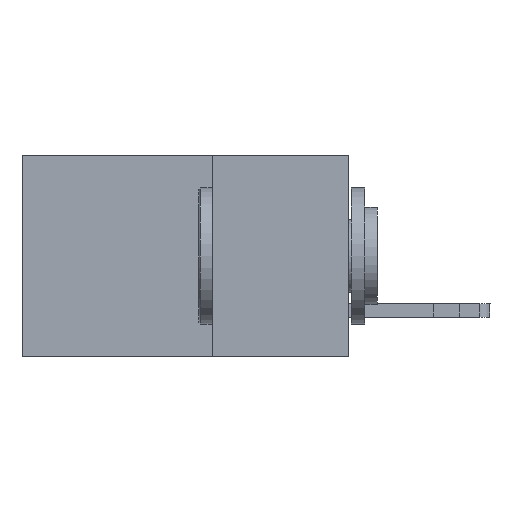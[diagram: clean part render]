
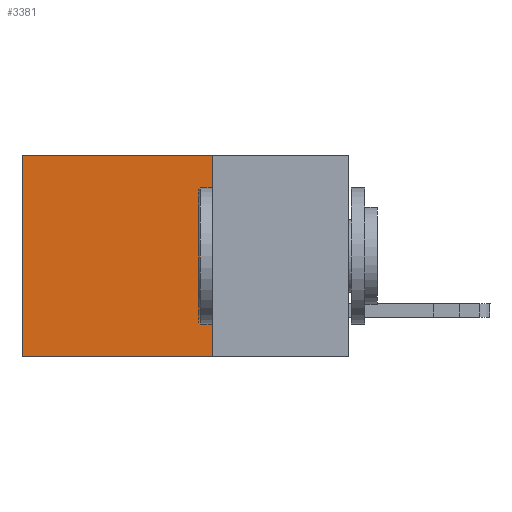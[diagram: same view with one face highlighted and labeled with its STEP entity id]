
A CAD part, left-side view. The second image highlights one B-rep face of the part: STEP entity #3381.
In plain terms, the highlighted planar face has unit normal (-1, 0, 0).
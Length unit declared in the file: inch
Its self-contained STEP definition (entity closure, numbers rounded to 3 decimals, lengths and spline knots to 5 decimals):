
#71 = CARTESIAN_POINT ( 'NONE',  ( 0.2615, 0.25, 0. ) ) ;
#159 = PLANE ( 'NONE',  #5733 ) ;
#172 = CARTESIAN_POINT ( 'NONE',  ( 0.2615, 0.25, -0.37 ) ) ;
#450 = ORIENTED_EDGE ( 'NONE', *, *, #9704, .T. ) ;
#469 = VERTEX_POINT ( 'NONE', #11647 ) ;
#1218 = VERTEX_POINT ( 'NONE', #1797 ) ;
#1279 = EDGE_LOOP ( 'NONE', ( #4782, #8911, #9141, #450 ) ) ;
#1305 = DIRECTION ( 'NONE',  ( 0., 0., -1. ) ) ;
#1797 = CARTESIAN_POINT ( 'NONE',  ( 0.2615, 0.25, -0.37 ) ) ;
#1915 = LINE ( 'NONE', #2898, #6736 ) ;
#2261 = LINE ( 'NONE', #172, #6209 ) ;
#2370 = DIRECTION ( 'NONE',  ( 0., 0., -1. ) ) ;
#2437 = VECTOR ( 'NONE', #9792, 39.37008 ) ;
#2898 = CARTESIAN_POINT ( 'NONE',  ( 0.2615, 0.6, -0.37 ) ) ;
#3381 = ADVANCED_FACE ( 'NONE', ( #3504 ), #159, .F. ) ;
#3504 = FACE_OUTER_BOUND ( 'NONE', #1279, .T. ) ;
#4010 = CARTESIAN_POINT ( 'NONE',  ( 0.2615, 0.6, 0. ) ) ;
#4064 = EDGE_CURVE ( 'NONE', #11904, #6744, #1915, .T. ) ;
#4187 = EDGE_CURVE ( 'NONE', #469, #1218, #2261, .T. ) ;
#4782 = ORIENTED_EDGE ( 'NONE', *, *, #4064, .T. ) ;
#5733 = AXIS2_PLACEMENT_3D ( 'NONE', #12101, #10030, #1305 ) ;
#6209 = VECTOR ( 'NONE', #2370, 39.37008 ) ;
#6217 = DIRECTION ( 'NONE',  ( 0., 0., -1. ) ) ;
#6736 = VECTOR ( 'NONE', #6217, 39.37008 ) ;
#6744 = VERTEX_POINT ( 'NONE', #8414 ) ;
#6995 = VECTOR ( 'NONE', #7631, 39.37008 ) ;
#7470 = EDGE_CURVE ( 'NONE', #1218, #6744, #13434, .T. ) ;
#7631 = DIRECTION ( 'NONE',  ( 0., 1., 0. ) ) ;
#8414 = CARTESIAN_POINT ( 'NONE',  ( 0.2615, 0.6, -0.37 ) ) ;
#8911 = ORIENTED_EDGE ( 'NONE', *, *, #7470, .F. ) ;
#9141 = ORIENTED_EDGE ( 'NONE', *, *, #4187, .F. ) ;
#9704 = EDGE_CURVE ( 'NONE', #469, #11904, #9904, .T. ) ;
#9792 = DIRECTION ( 'NONE',  ( 0., 1., 0. ) ) ;
#9904 = LINE ( 'NONE', #71, #6995 ) ;
#10030 = DIRECTION ( 'NONE',  ( 1., 0., 0. ) ) ;
#11647 = CARTESIAN_POINT ( 'NONE',  ( 0.2615, 0.25, 0. ) ) ;
#11904 = VERTEX_POINT ( 'NONE', #4010 ) ;
#12101 = CARTESIAN_POINT ( 'NONE',  ( 0.2615, 0.25, -0.37 ) ) ;
#12152 = CARTESIAN_POINT ( 'NONE',  ( 0.2615, 0.25, -0.37 ) ) ;
#13434 = LINE ( 'NONE', #12152, #2437 ) ;
